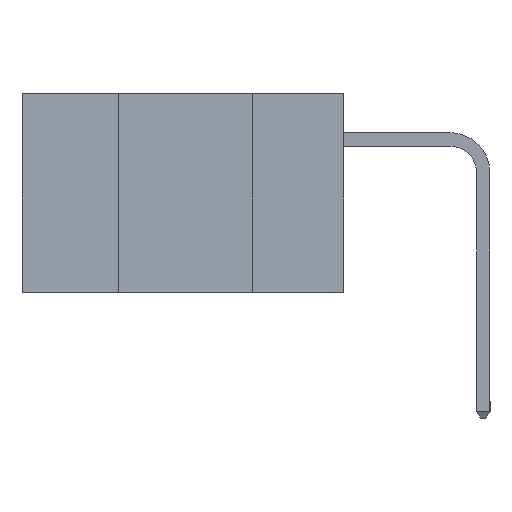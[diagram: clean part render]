
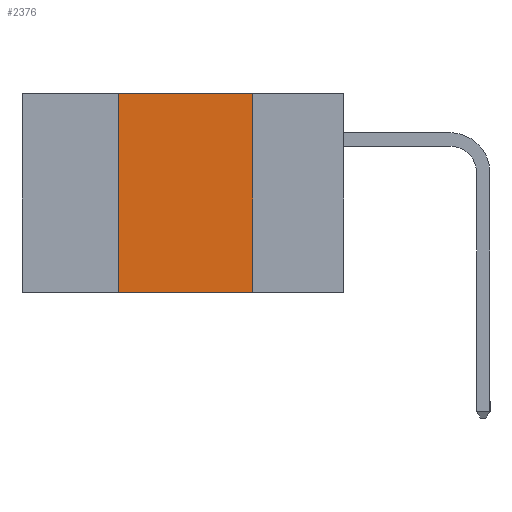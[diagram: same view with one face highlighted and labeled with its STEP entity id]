
A CAD part, left-side view. The second image highlights one B-rep face of the part: STEP entity #2376.
In plain terms, the highlighted planar face has unit normal (-1, 0, 0).
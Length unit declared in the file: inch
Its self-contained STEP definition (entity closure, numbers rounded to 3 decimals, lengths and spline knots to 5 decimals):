
#421 = EDGE_CURVE ( 'NONE', #7131, #6344, #19154, .T. ) ;
#475 = VECTOR ( 'NONE', #4167, 39.37008 ) ;
#968 = LINE ( 'NONE', #10377, #475 ) ;
#2376 = ADVANCED_FACE ( 'NONE', ( #19286 ), #12353, .F. ) ;
#2400 = ORIENTED_EDGE ( 'NONE', *, *, #421, .T. ) ;
#2537 = ORIENTED_EDGE ( 'NONE', *, *, #19474, .F. ) ;
#2566 = ORIENTED_EDGE ( 'NONE', *, *, #19237, .F. ) ;
#2759 = ORIENTED_EDGE ( 'NONE', *, *, #3062, .F. ) ;
#3062 = EDGE_CURVE ( 'NONE', #9706, #6344, #11282, .T. ) ;
#4167 = DIRECTION ( 'NONE',  ( 0., 0., 1. ) ) ;
#5860 = LINE ( 'NONE', #17055, #17923 ) ;
#6085 = CARTESIAN_POINT ( 'NONE',  ( 0., 0.17, -0.37 ) ) ;
#6344 = VERTEX_POINT ( 'NONE', #6085 ) ;
#6441 = DIRECTION ( 'NONE',  ( 0., 0., -1. ) ) ;
#6518 = CARTESIAN_POINT ( 'NONE',  ( 0., 0.17, -0.37 ) ) ;
#7131 = VERTEX_POINT ( 'NONE', #14085 ) ;
#7271 = VECTOR ( 'NONE', #12788, 39.37008 ) ;
#8037 = DIRECTION ( 'NONE',  ( 0., -1., 0. ) ) ;
#8259 = EDGE_LOOP ( 'NONE', ( #2759, #2566, #2537, #2400 ) ) ;
#9121 = AXIS2_PLACEMENT_3D ( 'NONE', #12189, #11919, #11918 ) ;
#9228 = VERTEX_POINT ( 'NONE', #18172 ) ;
#9706 = VERTEX_POINT ( 'NONE', #12800 ) ;
#10377 = CARTESIAN_POINT ( 'NONE',  ( 0., 0.42, -0.37 ) ) ;
#11282 = LINE ( 'NONE', #6518, #18635 ) ;
#11918 = DIRECTION ( 'NONE',  ( 0., 0., -1. ) ) ;
#11919 = DIRECTION ( 'NONE',  ( 1., 0., 0. ) ) ;
#12189 = CARTESIAN_POINT ( 'NONE',  ( 0., 0.6, 0. ) ) ;
#12353 = PLANE ( 'NONE',  #9121 ) ;
#12788 = DIRECTION ( 'NONE',  ( 0., -1., 0. ) ) ;
#12800 = CARTESIAN_POINT ( 'NONE',  ( 0., 0.17, 0. ) ) ;
#14085 = CARTESIAN_POINT ( 'NONE',  ( 0., 0.42, -0.37 ) ) ;
#17055 = CARTESIAN_POINT ( 'NONE',  ( 0., 0.6, 0. ) ) ;
#17571 = CARTESIAN_POINT ( 'NONE',  ( 0., 0.6, -0.37 ) ) ;
#17923 = VECTOR ( 'NONE', #8037, 39.37008 ) ;
#18172 = CARTESIAN_POINT ( 'NONE',  ( 0., 0.42, 0. ) ) ;
#18635 = VECTOR ( 'NONE', #6441, 39.37008 ) ;
#19154 = LINE ( 'NONE', #17571, #7271 ) ;
#19237 = EDGE_CURVE ( 'NONE', #9228, #9706, #5860, .T. ) ;
#19286 = FACE_OUTER_BOUND ( 'NONE', #8259, .T. ) ;
#19474 = EDGE_CURVE ( 'NONE', #7131, #9228, #968, .T. ) ;
